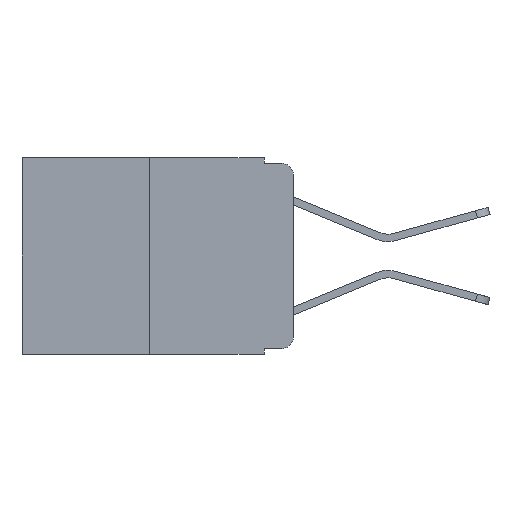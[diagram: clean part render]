
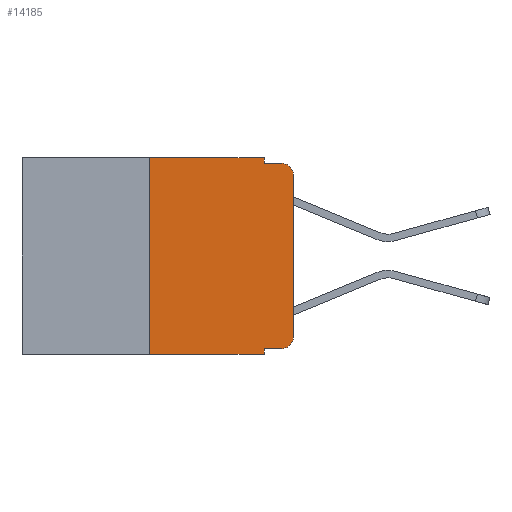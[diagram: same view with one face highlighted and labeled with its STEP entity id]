
A CAD part, left-side view. The second image highlights one B-rep face of the part: STEP entity #14185.
In plain terms, the highlighted planar face has unit normal (-1, 0, 0).
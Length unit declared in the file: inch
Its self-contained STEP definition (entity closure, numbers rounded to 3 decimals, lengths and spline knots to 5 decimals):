
#9 = VERTEX_POINT ( 'NONE', #239 ) ;
#239 = CARTESIAN_POINT ( 'NONE',  ( 0., 0.051, -0.343 ) ) ;
#479 = CARTESIAN_POINT ( 'NONE',  ( 0., 0., -0.03 ) ) ;
#577 = ORIENTED_EDGE ( 'NONE', *, *, #19796, .F. ) ;
#1001 = VERTEX_POINT ( 'NONE', #7205 ) ;
#1368 = DIRECTION ( 'NONE',  ( 0., -1., 0. ) ) ;
#1529 = VECTOR ( 'NONE', #7770, 39.37008 ) ;
#1636 = EDGE_CURVE ( 'NONE', #5405, #20491, #17943, .T. ) ;
#1661 = ORIENTED_EDGE ( 'NONE', *, *, #10545, .T. ) ;
#1801 = VERTEX_POINT ( 'NONE', #479 ) ;
#2010 = VERTEX_POINT ( 'NONE', #2177 ) ;
#2021 = DIRECTION ( 'NONE',  ( 0., -1., 0. ) ) ;
#2025 = CARTESIAN_POINT ( 'NONE',  ( 0., 0.051, 0. ) ) ;
#2177 = CARTESIAN_POINT ( 'NONE',  ( 0., 0.02, -0.333 ) ) ;
#2971 = CARTESIAN_POINT ( 'NONE',  ( 0., 0.051, -0.01 ) ) ;
#3137 = VERTEX_POINT ( 'NONE', #2025 ) ;
#3278 = DIRECTION ( 'NONE',  ( 0., 0., -1. ) ) ;
#3490 = ORIENTED_EDGE ( 'NONE', *, *, #18061, .T. ) ;
#3584 = VERTEX_POINT ( 'NONE', #15832 ) ;
#3753 = EDGE_CURVE ( 'NONE', #1801, #1001, #5402, .T. ) ;
#3776 = LINE ( 'NONE', #17833, #20001 ) ;
#4092 = VECTOR ( 'NONE', #6151, 39.37008 ) ;
#4317 = ORIENTED_EDGE ( 'NONE', *, *, #11398, .T. ) ;
#4507 = CARTESIAN_POINT ( 'NONE',  ( 0., 0., 0. ) ) ;
#5306 = VERTEX_POINT ( 'NONE', #11073 ) ;
#5402 = CIRCLE ( 'NONE', #13101, 0.02 ) ;
#5405 = VERTEX_POINT ( 'NONE', #14555 ) ;
#5467 = VECTOR ( 'NONE', #9170, 39.37008 ) ;
#6028 = DIRECTION ( 'NONE',  ( 1., 0., 0. ) ) ;
#6090 = ORIENTED_EDGE ( 'NONE', *, *, #13531, .F. ) ;
#6151 = DIRECTION ( 'NONE',  ( 0., 0., 1. ) ) ;
#6238 = CARTESIAN_POINT ( 'NONE',  ( 0., 0.051, 0. ) ) ;
#6646 = FACE_OUTER_BOUND ( 'NONE', #19745, .T. ) ;
#7205 = CARTESIAN_POINT ( 'NONE',  ( 0., 0.02, -0.01 ) ) ;
#7239 = CARTESIAN_POINT ( 'NONE',  ( 0., 0.473, -0.343 ) ) ;
#7770 = DIRECTION ( 'NONE',  ( 0., -1., 0. ) ) ;
#7939 = VERTEX_POINT ( 'NONE', #14227 ) ;
#8539 = VECTOR ( 'NONE', #17256, 39.37008 ) ;
#9148 = CARTESIAN_POINT ( 'NONE',  ( 0., 0.25, 0. ) ) ;
#9170 = DIRECTION ( 'NONE',  ( 0., 0., 1. ) ) ;
#9511 = CIRCLE ( 'NONE', #11484, 0.02 ) ;
#9613 = EDGE_CURVE ( 'NONE', #3137, #7939, #12727, .T. ) ;
#9751 = DIRECTION ( 'NONE',  ( -1., 0., 0. ) ) ;
#9853 = ORIENTED_EDGE ( 'NONE', *, *, #1636, .F. ) ;
#10545 = EDGE_CURVE ( 'NONE', #5405, #9, #19872, .T. ) ;
#10739 = CARTESIAN_POINT ( 'NONE',  ( 0., 0.051, 0. ) ) ;
#11073 = CARTESIAN_POINT ( 'NONE',  ( 0., 0.051, -0.333 ) ) ;
#11398 = EDGE_CURVE ( 'NONE', #5306, #2010, #14906, .T. ) ;
#11484 = AXIS2_PLACEMENT_3D ( 'NONE', #19015, #9751, #20482 ) ;
#11650 = LINE ( 'NONE', #10739, #14877 ) ;
#11686 = VECTOR ( 'NONE', #16633, 39.37008 ) ;
#12060 = ORIENTED_EDGE ( 'NONE', *, *, #3753, .T. ) ;
#12481 = EDGE_CURVE ( 'NONE', #2010, #3584, #9511, .T. ) ;
#12727 = LINE ( 'NONE', #6238, #8539 ) ;
#13101 = AXIS2_PLACEMENT_3D ( 'NONE', #19179, #18501, #3278 ) ;
#13531 = EDGE_CURVE ( 'NONE', #5306, #9, #11650, .T. ) ;
#14185 = ADVANCED_FACE ( 'NONE', ( #6646 ), #15510, .F. ) ;
#14227 = CARTESIAN_POINT ( 'NONE',  ( 0., 0.051, -0.01 ) ) ;
#14555 = CARTESIAN_POINT ( 'NONE',  ( 0., 0.25, -0.343 ) ) ;
#14877 = VECTOR ( 'NONE', #19954, 39.37008 ) ;
#14906 = LINE ( 'NONE', #15658, #1529 ) ;
#15472 = AXIS2_PLACEMENT_3D ( 'NONE', #19987, #6028, #16985 ) ;
#15510 = PLANE ( 'NONE',  #15472 ) ;
#15565 = VECTOR ( 'NONE', #1368, 39.37008 ) ;
#15658 = CARTESIAN_POINT ( 'NONE',  ( 0., 0.051, -0.333 ) ) ;
#15832 = CARTESIAN_POINT ( 'NONE',  ( 0., 0., -0.313 ) ) ;
#15916 = EDGE_CURVE ( 'NONE', #7939, #1001, #19562, .T. ) ;
#16633 = DIRECTION ( 'NONE',  ( 0., -1., 0. ) ) ;
#16645 = ORIENTED_EDGE ( 'NONE', *, *, #15916, .F. ) ;
#16718 = LINE ( 'NONE', #4507, #4092 ) ;
#16985 = DIRECTION ( 'NONE',  ( 0., 0., -1. ) ) ;
#17118 = ORIENTED_EDGE ( 'NONE', *, *, #9613, .F. ) ;
#17256 = DIRECTION ( 'NONE',  ( 0., 0., -1. ) ) ;
#17833 = CARTESIAN_POINT ( 'NONE',  ( 0., 0.473, 0. ) ) ;
#17943 = LINE ( 'NONE', #9148, #5467 ) ;
#18061 = EDGE_CURVE ( 'NONE', #3584, #1801, #16718, .T. ) ;
#18501 = DIRECTION ( 'NONE',  ( -1., 0., 0. ) ) ;
#18596 = ORIENTED_EDGE ( 'NONE', *, *, #12481, .T. ) ;
#19015 = CARTESIAN_POINT ( 'NONE',  ( 0., 0.02, -0.313 ) ) ;
#19179 = CARTESIAN_POINT ( 'NONE',  ( 0., 0.02, -0.03 ) ) ;
#19560 = CARTESIAN_POINT ( 'NONE',  ( 0., 0.25, 0. ) ) ;
#19562 = LINE ( 'NONE', #2971, #15565 ) ;
#19745 = EDGE_LOOP ( 'NONE', ( #3490, #12060, #16645, #17118, #577, #9853, #1661, #6090, #4317, #18596 ) ) ;
#19796 = EDGE_CURVE ( 'NONE', #20491, #3137, #3776, .T. ) ;
#19872 = LINE ( 'NONE', #7239, #11686 ) ;
#19954 = DIRECTION ( 'NONE',  ( 0., 0., -1. ) ) ;
#19987 = CARTESIAN_POINT ( 'NONE',  ( 0., 0.473, 0. ) ) ;
#20001 = VECTOR ( 'NONE', #2021, 39.37008 ) ;
#20482 = DIRECTION ( 'NONE',  ( 0., 0., -1. ) ) ;
#20491 = VERTEX_POINT ( 'NONE', #19560 ) ;
